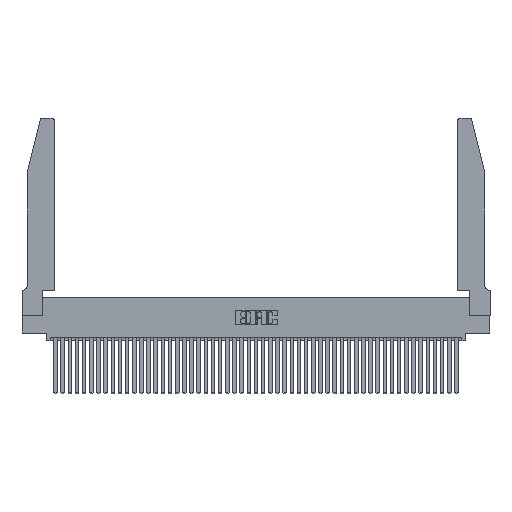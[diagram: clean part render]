
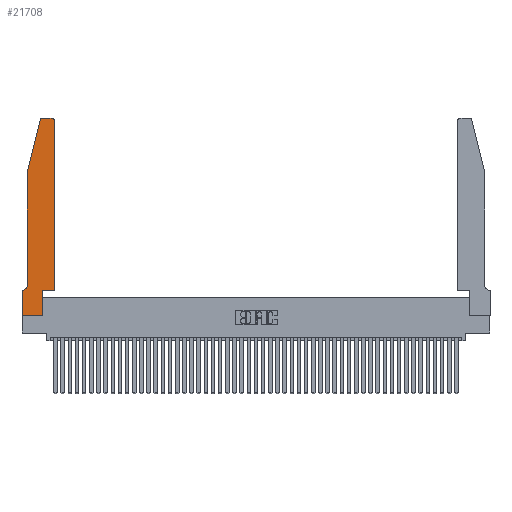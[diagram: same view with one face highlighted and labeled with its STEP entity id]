
A CAD part, top view. The second image highlights one B-rep face of the part: STEP entity #21708.
In plain terms, the highlighted planar face has unit normal (0, 0, 1).
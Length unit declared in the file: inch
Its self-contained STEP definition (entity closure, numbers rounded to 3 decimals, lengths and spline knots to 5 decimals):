
#128 = ORIENTED_EDGE ( 'NONE', *, *, #23046, .T. ) ;
#350 = CARTESIAN_POINT ( 'NONE',  ( 0.25487, 2.72718, 0.37 ) ) ;
#1263 = VERTEX_POINT ( 'NONE', #16815 ) ;
#1588 = CARTESIAN_POINT ( 'NONE',  ( 0.0755, 2., 0.37 ) ) ;
#1603 = DIRECTION ( 'NONE',  ( 1., 0., 0. ) ) ;
#1752 = CARTESIAN_POINT ( 'NONE',  ( 0., 0., 0.37 ) ) ;
#2369 = EDGE_CURVE ( 'NONE', #1263, #13417, #21943, .T. ) ;
#2902 = ORIENTED_EDGE ( 'NONE', *, *, #39128, .T. ) ;
#3044 = ORIENTED_EDGE ( 'NONE', *, *, #3815, .T. ) ;
#3371 = CARTESIAN_POINT ( 'NONE',  ( 0.0755, 0.42, 0.37 ) ) ;
#3583 = CARTESIAN_POINT ( 'NONE',  ( 0.0755, 2., 0.37 ) ) ;
#3815 = EDGE_CURVE ( 'NONE', #7930, #1263, #35615, .T. ) ;
#4350 = DIRECTION ( 'NONE',  ( 1., 0., 0. ) ) ;
#4523 = CARTESIAN_POINT ( 'NONE',  ( 0.284, 2.72, 0.37 ) ) ;
#4661 = ORIENTED_EDGE ( 'NONE', *, *, #34697, .T. ) ;
#4835 = AXIS2_PLACEMENT_3D ( 'NONE', #40818, #40660, #22594 ) ;
#4864 = DIRECTION ( 'NONE',  ( 0., -1., 0. ) ) ;
#5958 = CARTESIAN_POINT ( 'NONE',  ( 0., 0.35, 0.37 ) ) ;
#6602 = CARTESIAN_POINT ( 'NONE',  ( 0.2865, 0., 0.37 ) ) ;
#7370 = CARTESIAN_POINT ( 'NONE',  ( 0.4505, 2.72, 0.37 ) ) ;
#7472 = DIRECTION ( 'NONE',  ( 1., 0., 0. ) ) ;
#7684 = CARTESIAN_POINT ( 'NONE',  ( 0.0755, 0.35, 0.37 ) ) ;
#7725 = VECTOR ( 'NONE', #28262, 39.37008 ) ;
#7930 = VERTEX_POINT ( 'NONE', #32498 ) ;
#8570 = DIRECTION ( 'NONE',  ( 0., 1., 0. ) ) ;
#11329 = CARTESIAN_POINT ( 'NONE',  ( 0.4505, 0.35, 0.37 ) ) ;
#13417 = VERTEX_POINT ( 'NONE', #350 ) ;
#14845 = VERTEX_POINT ( 'NONE', #34189 ) ;
#14919 = VERTEX_POINT ( 'NONE', #5958 ) ;
#15673 = VECTOR ( 'NONE', #1603, 39.37008 ) ;
#16327 = DIRECTION ( 'NONE',  ( 0., 0., -1. ) ) ;
#16815 = CARTESIAN_POINT ( 'NONE',  ( 0.284, 2.75, 0.37 ) ) ;
#18094 = LINE ( 'NONE', #26110, #22088 ) ;
#18920 = VERTEX_POINT ( 'NONE', #46998 ) ;
#19826 = VECTOR ( 'NONE', #4864, 39.37008 ) ;
#20667 = ORIENTED_EDGE ( 'NONE', *, *, #36118, .T. ) ;
#21070 = CARTESIAN_POINT ( 'NONE',  ( 0.0755, 2., 0.37 ) ) ;
#21708 = ADVANCED_FACE ( 'NONE', ( #42844 ), #37455, .T. ) ;
#21943 = CIRCLE ( 'NONE', #35700, 0.03 ) ;
#22063 = ORIENTED_EDGE ( 'NONE', *, *, #46721, .T. ) ;
#22088 = VECTOR ( 'NONE', #28651, 39.37008 ) ;
#22594 = DIRECTION ( 'NONE',  ( 1., 0., 0. ) ) ;
#23046 = EDGE_CURVE ( 'NONE', #14919, #43001, #45584, .T. ) ;
#23438 = EDGE_LOOP ( 'NONE', ( #3044, #38234, #29784, #20667, #22063, #41469, #128, #26727, #42667, #2902, #30617, #4661 ) ) ;
#23686 = EDGE_CURVE ( 'NONE', #14845, #14919, #26125, .T. ) ;
#23749 = VERTEX_POINT ( 'NONE', #1588 ) ;
#25633 = EDGE_CURVE ( 'NONE', #13417, #23749, #31663, .T. ) ;
#26110 = CARTESIAN_POINT ( 'NONE',  ( 0.2865, 0.35, 0.37 ) ) ;
#26125 = LINE ( 'NONE', #7684, #31267 ) ;
#26310 = DIRECTION ( 'NONE',  ( 0., 0., 1. ) ) ;
#26327 = CARTESIAN_POINT ( 'NONE',  ( 0., 0., 0.37 ) ) ;
#26727 = ORIENTED_EDGE ( 'NONE', *, *, #42360, .T. ) ;
#26927 = LINE ( 'NONE', #11329, #35501 ) ;
#27210 = CARTESIAN_POINT ( 'NONE',  ( 0.0055, 0.42, 0.37 ) ) ;
#27363 = VERTEX_POINT ( 'NONE', #41298 ) ;
#27369 = AXIS2_PLACEMENT_3D ( 'NONE', #27210, #16327, #34094 ) ;
#28262 = DIRECTION ( 'NONE',  ( 0., -1., 0. ) ) ;
#28651 = DIRECTION ( 'NONE',  ( 0., 1., 0. ) ) ;
#29784 = ORIENTED_EDGE ( 'NONE', *, *, #25633, .T. ) ;
#30085 = CARTESIAN_POINT ( 'NONE',  ( 0.2605, 2.75, 0.37 ) ) ;
#30165 = CIRCLE ( 'NONE', #39614, 0.03 ) ;
#30171 = DIRECTION ( 'NONE',  ( 0., 0., 1. ) ) ;
#30617 = ORIENTED_EDGE ( 'NONE', *, *, #33425, .T. ) ;
#31075 = CIRCLE ( 'NONE', #27369, 0.07 ) ;
#31103 = LINE ( 'NONE', #1752, #15673 ) ;
#31267 = VECTOR ( 'NONE', #40523, 39.37008 ) ;
#31663 = LINE ( 'NONE', #3583, #45397 ) ;
#32498 = CARTESIAN_POINT ( 'NONE',  ( 0.4205, 2.75, 0.37 ) ) ;
#33137 = VECTOR ( 'NONE', #8570, 39.37008 ) ;
#33425 = EDGE_CURVE ( 'NONE', #27363, #42021, #40022, .T. ) ;
#34094 = DIRECTION ( 'NONE',  ( -1., 0., 0. ) ) ;
#34189 = CARTESIAN_POINT ( 'NONE',  ( 0.0055, 0.35, 0.37 ) ) ;
#34299 = CARTESIAN_POINT ( 'NONE',  ( 0.4205, 2.72, 0.37 ) ) ;
#34381 = CARTESIAN_POINT ( 'NONE',  ( 0.4505, 0.35, 0.37 ) ) ;
#34697 = EDGE_CURVE ( 'NONE', #42021, #7930, #30165, .T. ) ;
#34986 = EDGE_CURVE ( 'NONE', #36196, #18920, #18094, .T. ) ;
#35501 = VECTOR ( 'NONE', #7472, 39.37008 ) ;
#35615 = LINE ( 'NONE', #30085, #38447 ) ;
#35700 = AXIS2_PLACEMENT_3D ( 'NONE', #4523, #30171, #41810 ) ;
#36118 = EDGE_CURVE ( 'NONE', #23749, #39624, #46092, .T. ) ;
#36196 = VERTEX_POINT ( 'NONE', #6602 ) ;
#37455 = PLANE ( 'NONE',  #4835 ) ;
#37839 = CARTESIAN_POINT ( 'NONE',  ( 0., 0., 0.37 ) ) ;
#38234 = ORIENTED_EDGE ( 'NONE', *, *, #2369, .T. ) ;
#38447 = VECTOR ( 'NONE', #45282, 39.37008 ) ;
#39128 = EDGE_CURVE ( 'NONE', #18920, #27363, #26927, .T. ) ;
#39614 = AXIS2_PLACEMENT_3D ( 'NONE', #34299, #26310, #4350 ) ;
#39624 = VERTEX_POINT ( 'NONE', #3371 ) ;
#40022 = LINE ( 'NONE', #34381, #33137 ) ;
#40523 = DIRECTION ( 'NONE',  ( -1., 0., 0. ) ) ;
#40660 = DIRECTION ( 'NONE',  ( 0., 0., 1. ) ) ;
#40818 = CARTESIAN_POINT ( 'NONE',  ( 0., 0.35, 0.37 ) ) ;
#41298 = CARTESIAN_POINT ( 'NONE',  ( 0.4505, 0.35, 0.37 ) ) ;
#41469 = ORIENTED_EDGE ( 'NONE', *, *, #23686, .T. ) ;
#41810 = DIRECTION ( 'NONE',  ( 1., 0., 0. ) ) ;
#42021 = VERTEX_POINT ( 'NONE', #7370 ) ;
#42360 = EDGE_CURVE ( 'NONE', #43001, #36196, #31103, .T. ) ;
#42667 = ORIENTED_EDGE ( 'NONE', *, *, #34986, .T. ) ;
#42844 = FACE_OUTER_BOUND ( 'NONE', #23438, .T. ) ;
#43001 = VERTEX_POINT ( 'NONE', #26327 ) ;
#43788 = DIRECTION ( 'NONE',  ( -0.239, -0.971, 0. ) ) ;
#45282 = DIRECTION ( 'NONE',  ( -1., 0., 0. ) ) ;
#45397 = VECTOR ( 'NONE', #43788, 39.37008 ) ;
#45584 = LINE ( 'NONE', #37839, #19826 ) ;
#46092 = LINE ( 'NONE', #21070, #7725 ) ;
#46721 = EDGE_CURVE ( 'NONE', #39624, #14845, #31075, .T. ) ;
#46998 = CARTESIAN_POINT ( 'NONE',  ( 0.2865, 0.35, 0.37 ) ) ;
